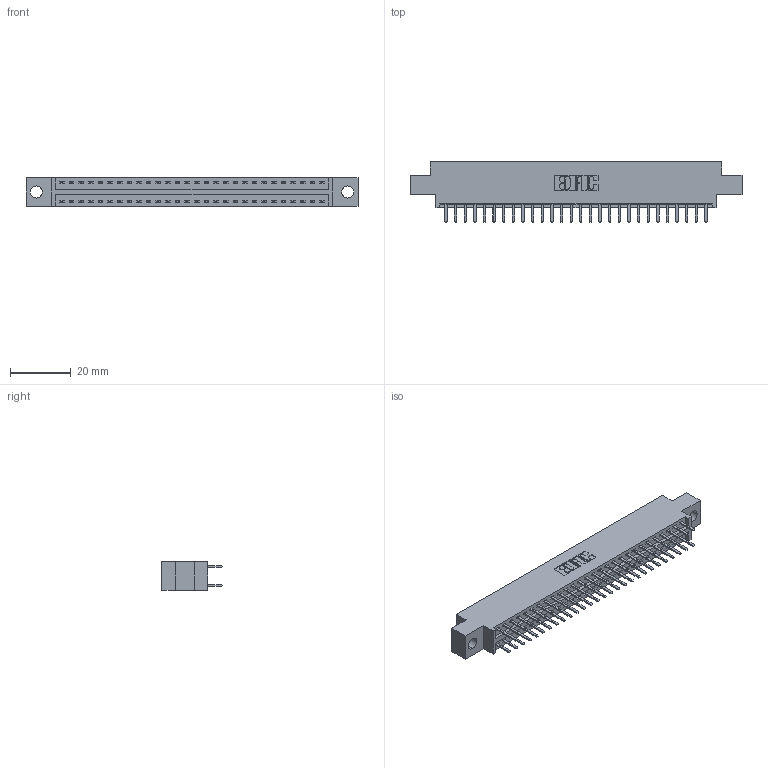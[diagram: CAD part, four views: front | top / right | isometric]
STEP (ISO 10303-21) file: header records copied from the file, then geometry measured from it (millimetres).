
FILE_DESCRIPTION (( 'STEP AP203' ), '1' );
FILE_NAME ('346-056-520-804.STEP', '2022-05-21T05:05:20', ( '' ), ( '' ), 'SwSTEP 2.0', 'SolidWorks 2020', '' );
FILE_SCHEMA (( 'CONFIG_CONTROL_DESIGN' ));
Length unit declared in the file: inch
Products named in the file (3): 346-056-520-804; 346 Part_0.170 Offset - 0.156 Dia-TH; 345-292-001_345-293-120
Assembly tree (57 placements, depth 2):
  346-056-520-804
    346 Part_0.170 Offset - 0.156 Dia-TH
    345-292-001_345-293-120  x56
Bounding box: 109.47 x 20.02 x 9.4 mm (x, y, z)
Volume: 10281.2 mm3; surface area: 13881.9 mm2
Topology: 57 solids, 57 shells, 3276 faces, 9505 edges, 6186 vertices
Faces by surface type: plane 2166, cylinder 1110
Entity records: 20823 total; most frequent: CARTESIAN_POINT 3470, ORIENTED_EDGE 3390, DIRECTION 3095, EDGE_CURVE 1695, VECTOR 1447, LINE 1447, VERTEX_POINT 1126, AXIS2_PLACEMENT_3D 824
